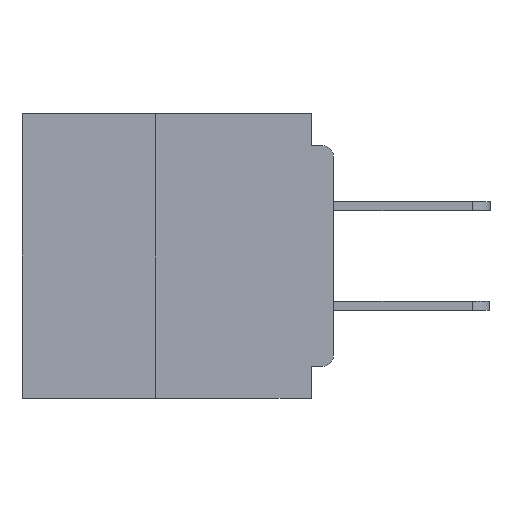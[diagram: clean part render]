
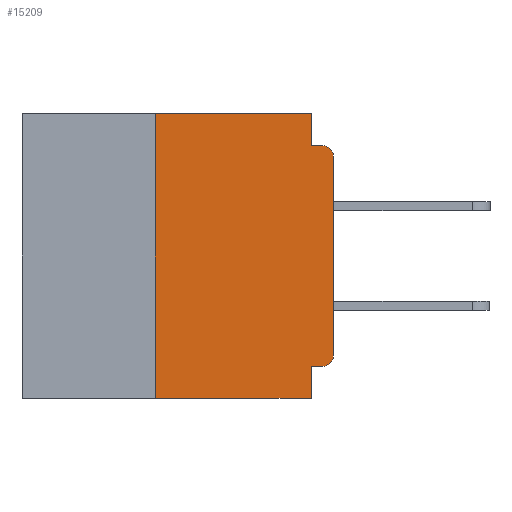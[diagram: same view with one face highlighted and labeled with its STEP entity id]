
A CAD part, left-side view. The second image highlights one B-rep face of the part: STEP entity #15209.
In plain terms, the highlighted planar face has unit normal (-1, 0, 0).
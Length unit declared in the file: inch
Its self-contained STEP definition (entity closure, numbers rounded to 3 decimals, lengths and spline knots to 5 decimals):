
#730 = DIRECTION ( 'NONE',  ( -1., 0., 0. ) ) ;
#1208 = VECTOR ( 'NONE', #32798, 39.37008 ) ;
#1255 = ORIENTED_EDGE ( 'NONE', *, *, #9551, .F. ) ;
#2074 = EDGE_CURVE ( 'NONE', #28232, #11593, #7511, .T. ) ;
#2208 = VERTEX_POINT ( 'NONE', #13664 ) ;
#3121 = CARTESIAN_POINT ( 'NONE',  ( 0., 0.437, 0. ) ) ;
#5308 = VERTEX_POINT ( 'NONE', #24833 ) ;
#5591 = ORIENTED_EDGE ( 'NONE', *, *, #17239, .T. ) ;
#5604 = VERTEX_POINT ( 'NONE', #8123 ) ;
#6184 = VECTOR ( 'NONE', #35105, 39.37008 ) ;
#6474 = DIRECTION ( 'NONE',  ( 0., 0., -1. ) ) ;
#7247 = CARTESIAN_POINT ( 'NONE',  ( 0., 0.015, -0.045 ) ) ;
#7511 = LINE ( 'NONE', #20093, #36159 ) ;
#7603 = CARTESIAN_POINT ( 'NONE',  ( 0., 0., -0.06 ) ) ;
#7996 = CARTESIAN_POINT ( 'NONE',  ( 0., 0.031, 0. ) ) ;
#8123 = CARTESIAN_POINT ( 'NONE',  ( 0., 0.25, -0.4 ) ) ;
#8642 = VERTEX_POINT ( 'NONE', #24099 ) ;
#8664 = LINE ( 'NONE', #21607, #1208 ) ;
#9311 = CIRCLE ( 'NONE', #34520, 0.015 ) ;
#9551 = EDGE_CURVE ( 'NONE', #5308, #29107, #34263, .T. ) ;
#9979 = CARTESIAN_POINT ( 'NONE',  ( 0., 0.437, 0. ) ) ;
#10264 = EDGE_CURVE ( 'NONE', #5604, #5308, #25506, .T. ) ;
#10383 = CARTESIAN_POINT ( 'NONE',  ( 0., 0.015, -0.06 ) ) ;
#10448 = LINE ( 'NONE', #7996, #24426 ) ;
#11437 = VERTEX_POINT ( 'NONE', #35857 ) ;
#11593 = VERTEX_POINT ( 'NONE', #28285 ) ;
#11679 = EDGE_CURVE ( 'NONE', #11437, #8642, #9311, .T. ) ;
#12455 = ORIENTED_EDGE ( 'NONE', *, *, #33536, .F. ) ;
#12992 = ORIENTED_EDGE ( 'NONE', *, *, #28699, .F. ) ;
#13319 = DIRECTION ( 'NONE',  ( 0., 0., -1. ) ) ;
#13664 = CARTESIAN_POINT ( 'NONE',  ( 0., 0.031, -0.045 ) ) ;
#13691 = LINE ( 'NONE', #32234, #6184 ) ;
#13707 = DIRECTION ( 'NONE',  ( 0., 0., 1. ) ) ;
#13756 = ORIENTED_EDGE ( 'NONE', *, *, #2074, .F. ) ;
#15209 = ADVANCED_FACE ( 'NONE', ( #33019 ), #24122, .F. ) ;
#15927 = DIRECTION ( 'NONE',  ( 0., 0., -1. ) ) ;
#16103 = CARTESIAN_POINT ( 'NONE',  ( 0., 0.031, -0.355 ) ) ;
#16770 = CIRCLE ( 'NONE', #28845, 0.015 ) ;
#17239 = EDGE_CURVE ( 'NONE', #24787, #19885, #16770, .T. ) ;
#17600 = CARTESIAN_POINT ( 'NONE',  ( 0., 0.015, -0.34 ) ) ;
#17708 = EDGE_LOOP ( 'NONE', ( #28347, #5591, #12455, #26601, #1255, #25317, #21629, #13756, #12992, #19204 ) ) ;
#18167 = VECTOR ( 'NONE', #13707, 39.37008 ) ;
#18605 = CARTESIAN_POINT ( 'NONE',  ( 0., 0., -0.355 ) ) ;
#19204 = ORIENTED_EDGE ( 'NONE', *, *, #11679, .T. ) ;
#19662 = DIRECTION ( 'NONE',  ( 0., -1., 0. ) ) ;
#19885 = VERTEX_POINT ( 'NONE', #7247 ) ;
#20093 = CARTESIAN_POINT ( 'NONE',  ( 0., 0.031, -0.4 ) ) ;
#20349 = DIRECTION ( 'NONE',  ( 0., 0., -1. ) ) ;
#20475 = LINE ( 'NONE', #34785, #34395 ) ;
#20926 = DIRECTION ( 'NONE',  ( 0., 0., 1. ) ) ;
#21607 = CARTESIAN_POINT ( 'NONE',  ( 0., 0., -0.045 ) ) ;
#21629 = ORIENTED_EDGE ( 'NONE', *, *, #31621, .T. ) ;
#23022 = CARTESIAN_POINT ( 'NONE',  ( 0., 0.031, 0. ) ) ;
#23328 = EDGE_CURVE ( 'NONE', #29107, #2208, #10448, .T. ) ;
#24099 = CARTESIAN_POINT ( 'NONE',  ( 0., 0., -0.34 ) ) ;
#24122 = PLANE ( 'NONE',  #33647 ) ;
#24426 = VECTOR ( 'NONE', #24695, 39.37008 ) ;
#24695 = DIRECTION ( 'NONE',  ( 0., 0., -1. ) ) ;
#24787 = VERTEX_POINT ( 'NONE', #7603 ) ;
#24833 = CARTESIAN_POINT ( 'NONE',  ( 0., 0.25, 0. ) ) ;
#25317 = ORIENTED_EDGE ( 'NONE', *, *, #10264, .F. ) ;
#25506 = LINE ( 'NONE', #30192, #18167 ) ;
#26601 = ORIENTED_EDGE ( 'NONE', *, *, #23328, .F. ) ;
#26979 = DIRECTION ( 'NONE',  ( 0., 1., 0. ) ) ;
#28232 = VERTEX_POINT ( 'NONE', #16103 ) ;
#28285 = CARTESIAN_POINT ( 'NONE',  ( 0., 0.031, -0.4 ) ) ;
#28347 = ORIENTED_EDGE ( 'NONE', *, *, #32782, .T. ) ;
#28699 = EDGE_CURVE ( 'NONE', #11437, #28232, #30839, .T. ) ;
#28845 = AXIS2_PLACEMENT_3D ( 'NONE', #10383, #29927, #13319 ) ;
#29107 = VERTEX_POINT ( 'NONE', #23022 ) ;
#29927 = DIRECTION ( 'NONE',  ( -1., 0., 0. ) ) ;
#29966 = VECTOR ( 'NONE', #26979, 39.37008 ) ;
#30192 = CARTESIAN_POINT ( 'NONE',  ( 0., 0.25, -0.4 ) ) ;
#30839 = LINE ( 'NONE', #18605, #29966 ) ;
#31621 = EDGE_CURVE ( 'NONE', #5604, #11593, #13691, .T. ) ;
#32234 = CARTESIAN_POINT ( 'NONE',  ( 0., 0.437, -0.4 ) ) ;
#32523 = DIRECTION ( 'NONE',  ( 1., 0., 0. ) ) ;
#32782 = EDGE_CURVE ( 'NONE', #8642, #24787, #20475, .T. ) ;
#32798 = DIRECTION ( 'NONE',  ( 0., -1., 0. ) ) ;
#33019 = FACE_OUTER_BOUND ( 'NONE', #17708, .T. ) ;
#33536 = EDGE_CURVE ( 'NONE', #2208, #19885, #8664, .T. ) ;
#33647 = AXIS2_PLACEMENT_3D ( 'NONE', #9979, #32523, #15927 ) ;
#34263 = LINE ( 'NONE', #3121, #35938 ) ;
#34395 = VECTOR ( 'NONE', #20926, 39.37008 ) ;
#34520 = AXIS2_PLACEMENT_3D ( 'NONE', #17600, #730, #20349 ) ;
#34785 = CARTESIAN_POINT ( 'NONE',  ( 0., 0., 0. ) ) ;
#35105 = DIRECTION ( 'NONE',  ( 0., -1., 0. ) ) ;
#35857 = CARTESIAN_POINT ( 'NONE',  ( 0., 0.015, -0.355 ) ) ;
#35938 = VECTOR ( 'NONE', #19662, 39.37008 ) ;
#36159 = VECTOR ( 'NONE', #6474, 39.37008 ) ;
